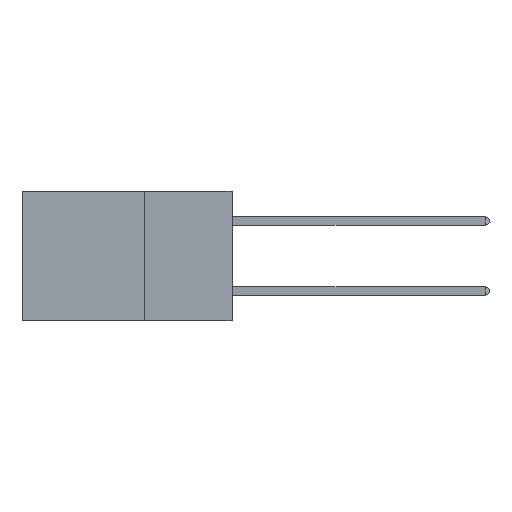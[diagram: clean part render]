
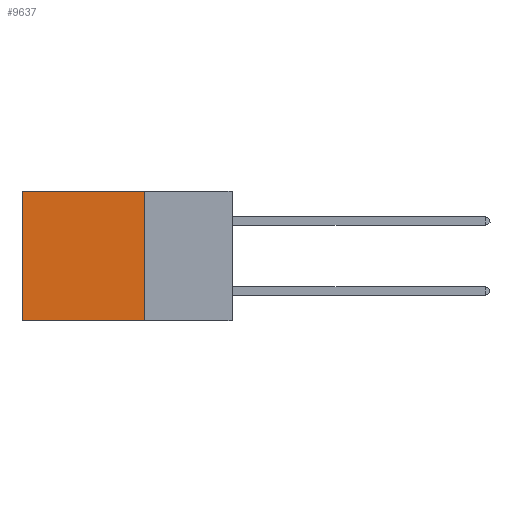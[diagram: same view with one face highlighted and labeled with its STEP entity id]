
A CAD part, left-side view. The second image highlights one B-rep face of the part: STEP entity #9637.
In plain terms, the highlighted planar face has unit normal (-1, 0, 0).
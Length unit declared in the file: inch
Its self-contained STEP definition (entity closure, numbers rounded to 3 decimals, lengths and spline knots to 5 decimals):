
#693 = ORIENTED_EDGE ( 'NONE', *, *, #1696, .F. ) ;
#1172 = ORIENTED_EDGE ( 'NONE', *, *, #14415, .F. ) ;
#1292 = DIRECTION ( 'NONE',  ( 0., 1., 0. ) ) ;
#1696 = EDGE_CURVE ( 'NONE', #16578, #3168, #7621, .T. ) ;
#2260 = LINE ( 'NONE', #9230, #4863 ) ;
#2407 = DIRECTION ( 'NONE',  ( 1., 0., 0. ) ) ;
#3168 = VERTEX_POINT ( 'NONE', #13138 ) ;
#3488 = VERTEX_POINT ( 'NONE', #10983 ) ;
#3867 = PLANE ( 'NONE',  #13542 ) ;
#4150 = EDGE_LOOP ( 'NONE', ( #6699, #693, #1172, #17578 ) ) ;
#4863 = VECTOR ( 'NONE', #15599, 39.37008 ) ;
#5170 = CARTESIAN_POINT ( 'NONE',  ( 0.2875, 0.6, 0. ) ) ;
#5519 = DIRECTION ( 'NONE',  ( 0., 0., -1. ) ) ;
#5645 = DIRECTION ( 'NONE',  ( 0., 1., 0. ) ) ;
#5900 = VECTOR ( 'NONE', #10177, 39.37008 ) ;
#6206 = LINE ( 'NONE', #9113, #13535 ) ;
#6245 = EDGE_CURVE ( 'NONE', #3488, #16428, #6206, .T. ) ;
#6699 = ORIENTED_EDGE ( 'NONE', *, *, #19181, .T. ) ;
#7621 = LINE ( 'NONE', #15246, #19505 ) ;
#9113 = CARTESIAN_POINT ( 'NONE',  ( 0.2875, 0.25, 0. ) ) ;
#9230 = CARTESIAN_POINT ( 'NONE',  ( 0.2875, 0.25, 0. ) ) ;
#9637 = ADVANCED_FACE ( 'NONE', ( #18464 ), #3867, .F. ) ;
#10177 = DIRECTION ( 'NONE',  ( 0., 0., -1. ) ) ;
#10983 = CARTESIAN_POINT ( 'NONE',  ( 0.2875, 0.25, 0. ) ) ;
#11882 = CARTESIAN_POINT ( 'NONE',  ( 0.2875, 0.6, 0. ) ) ;
#13138 = CARTESIAN_POINT ( 'NONE',  ( 0.2875, 0.6, -0.37 ) ) ;
#13460 = LINE ( 'NONE', #11882, #5900 ) ;
#13535 = VECTOR ( 'NONE', #1292, 39.37008 ) ;
#13542 = AXIS2_PLACEMENT_3D ( 'NONE', #18399, #2407, #5519 ) ;
#14415 = EDGE_CURVE ( 'NONE', #3488, #16578, #2260, .T. ) ;
#15246 = CARTESIAN_POINT ( 'NONE',  ( 0.2875, 0.25, -0.37 ) ) ;
#15599 = DIRECTION ( 'NONE',  ( 0., 0., -1. ) ) ;
#16428 = VERTEX_POINT ( 'NONE', #5170 ) ;
#16578 = VERTEX_POINT ( 'NONE', #20351 ) ;
#17578 = ORIENTED_EDGE ( 'NONE', *, *, #6245, .T. ) ;
#18399 = CARTESIAN_POINT ( 'NONE',  ( 0.2875, 0.25, 0. ) ) ;
#18464 = FACE_OUTER_BOUND ( 'NONE', #4150, .T. ) ;
#19181 = EDGE_CURVE ( 'NONE', #16428, #3168, #13460, .T. ) ;
#19505 = VECTOR ( 'NONE', #5645, 39.37008 ) ;
#20351 = CARTESIAN_POINT ( 'NONE',  ( 0.2875, 0.25, -0.37 ) ) ;
